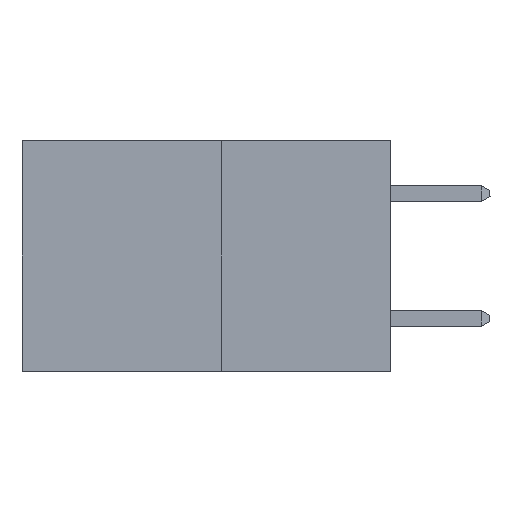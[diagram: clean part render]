
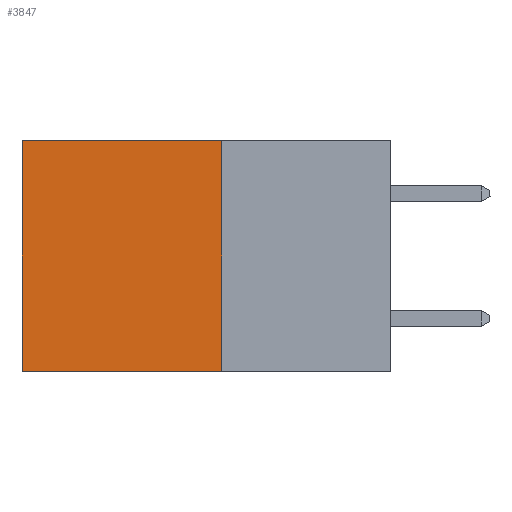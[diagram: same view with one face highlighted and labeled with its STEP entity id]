
A CAD part, left-side view. The second image highlights one B-rep face of the part: STEP entity #3847.
In plain terms, the highlighted planar face has unit normal (-1, 0, 0).
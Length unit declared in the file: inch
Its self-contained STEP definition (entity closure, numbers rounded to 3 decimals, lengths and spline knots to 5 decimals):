
#163 = AXIS2_PLACEMENT_3D ( 'NONE', #3712, #705, #316 ) ;
#316 = DIRECTION ( 'NONE',  ( 0., 0., -1. ) ) ;
#576 = VECTOR ( 'NONE', #10558, 39.37008 ) ;
#705 = DIRECTION ( 'NONE',  ( 1., 0., 0. ) ) ;
#829 = VECTOR ( 'NONE', #2641, 39.37008 ) ;
#1302 = PLANE ( 'NONE',  #163 ) ;
#1908 = CARTESIAN_POINT ( 'NONE',  ( 0.277, 0.27, 0. ) ) ;
#1943 = DIRECTION ( 'NONE',  ( 0., 1., 0. ) ) ;
#2246 = EDGE_CURVE ( 'NONE', #10553, #9237, #8708, .T. ) ;
#2546 = FACE_OUTER_BOUND ( 'NONE', #10236, .T. ) ;
#2641 = DIRECTION ( 'NONE',  ( 0., 0., -1. ) ) ;
#2810 = LINE ( 'NONE', #7025, #576 ) ;
#3712 = CARTESIAN_POINT ( 'NONE',  ( 0.277, 0.27, -0.37 ) ) ;
#3847 = ADVANCED_FACE ( 'NONE', ( #2546 ), #1302, .F. ) ;
#4287 = ORIENTED_EDGE ( 'NONE', *, *, #2246, .T. ) ;
#4331 = VERTEX_POINT ( 'NONE', #9665 ) ;
#4416 = ORIENTED_EDGE ( 'NONE', *, *, #6225, .F. ) ;
#4438 = CARTESIAN_POINT ( 'NONE',  ( 0.277, 0.27, -0.37 ) ) ;
#4500 = ORIENTED_EDGE ( 'NONE', *, *, #4824, .F. ) ;
#4824 = EDGE_CURVE ( 'NONE', #5627, #4331, #10799, .T. ) ;
#5016 = ORIENTED_EDGE ( 'NONE', *, *, #7567, .T. ) ;
#5627 = VERTEX_POINT ( 'NONE', #11553 ) ;
#6074 = LINE ( 'NONE', #8071, #829 ) ;
#6225 = EDGE_CURVE ( 'NONE', #10553, #5627, #2810, .T. ) ;
#6390 = VECTOR ( 'NONE', #9782, 39.37008 ) ;
#7025 = CARTESIAN_POINT ( 'NONE',  ( 0.277, 0.27, -0.37 ) ) ;
#7567 = EDGE_CURVE ( 'NONE', #9237, #4331, #6074, .T. ) ;
#8064 = CARTESIAN_POINT ( 'NONE',  ( 0.277, 0.27, 0. ) ) ;
#8071 = CARTESIAN_POINT ( 'NONE',  ( 0.277, 0.59, -0.37 ) ) ;
#8708 = LINE ( 'NONE', #8064, #10737 ) ;
#9237 = VERTEX_POINT ( 'NONE', #9244 ) ;
#9244 = CARTESIAN_POINT ( 'NONE',  ( 0.277, 0.59, 0. ) ) ;
#9665 = CARTESIAN_POINT ( 'NONE',  ( 0.277, 0.59, -0.37 ) ) ;
#9782 = DIRECTION ( 'NONE',  ( 0., 1., 0. ) ) ;
#10236 = EDGE_LOOP ( 'NONE', ( #5016, #4500, #4416, #4287 ) ) ;
#10553 = VERTEX_POINT ( 'NONE', #1908 ) ;
#10558 = DIRECTION ( 'NONE',  ( 0., 0., -1. ) ) ;
#10737 = VECTOR ( 'NONE', #1943, 39.37008 ) ;
#10799 = LINE ( 'NONE', #4438, #6390 ) ;
#11553 = CARTESIAN_POINT ( 'NONE',  ( 0.277, 0.27, -0.37 ) ) ;
